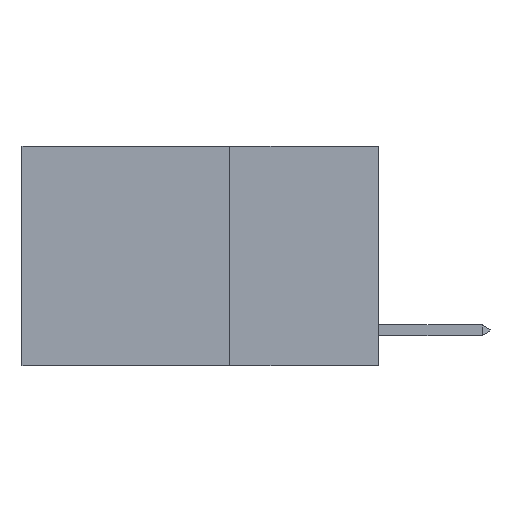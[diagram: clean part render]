
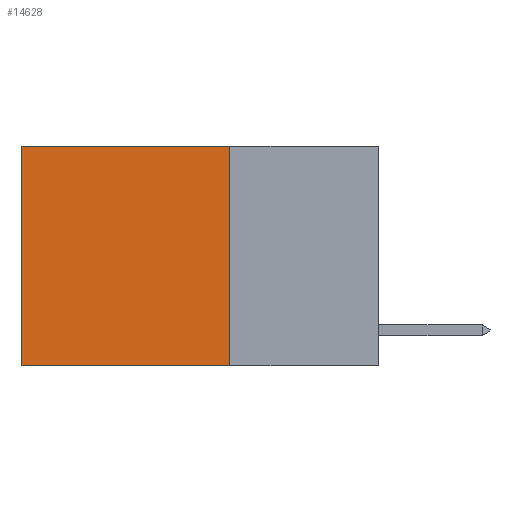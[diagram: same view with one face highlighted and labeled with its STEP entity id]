
A CAD part, left-side view. The second image highlights one B-rep face of the part: STEP entity #14628.
In plain terms, the highlighted planar face has unit normal (-1, 0, 0).
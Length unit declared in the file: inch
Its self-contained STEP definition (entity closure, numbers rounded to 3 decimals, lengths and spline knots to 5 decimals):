
#50 = CARTESIAN_POINT ( 'NONE',  ( 0.2625, 0.25, 0. ) ) ;
#1735 = EDGE_CURVE ( 'NONE', #9498, #5175, #27123, .T. ) ;
#2881 = ORIENTED_EDGE ( 'NONE', *, *, #27607, .F. ) ;
#4016 = EDGE_LOOP ( 'NONE', ( #20847, #16094, #2881, #5818 ) ) ;
#5175 = VERTEX_POINT ( 'NONE', #7162 ) ;
#5801 = CARTESIAN_POINT ( 'NONE',  ( 0.2625, 0.25, 0. ) ) ;
#5818 = ORIENTED_EDGE ( 'NONE', *, *, #21517, .T. ) ;
#5826 = EDGE_CURVE ( 'NONE', #18663, #5175, #27800, .T. ) ;
#7162 = CARTESIAN_POINT ( 'NONE',  ( 0.2625, 0.6, -0.37 ) ) ;
#7551 = DIRECTION ( 'NONE',  ( 0., 0., -1. ) ) ;
#7952 = PLANE ( 'NONE',  #23879 ) ;
#7965 = VERTEX_POINT ( 'NONE', #22360 ) ;
#9435 = VECTOR ( 'NONE', #19417, 39.37008 ) ;
#9498 = VERTEX_POINT ( 'NONE', #12818 ) ;
#9858 = CARTESIAN_POINT ( 'NONE',  ( 0.2625, 0.25, 0. ) ) ;
#10799 = LINE ( 'NONE', #50, #9435 ) ;
#11906 = CARTESIAN_POINT ( 'NONE',  ( 0.2625, 0.6, 0. ) ) ;
#12309 = DIRECTION ( 'NONE',  ( 0., 0., -1. ) ) ;
#12818 = CARTESIAN_POINT ( 'NONE',  ( 0.2625, 0.6, 0. ) ) ;
#14628 = ADVANCED_FACE ( 'NONE', ( #20873 ), #7952, .F. ) ;
#15901 = DIRECTION ( 'NONE',  ( 0., 1., 0. ) ) ;
#16094 = ORIENTED_EDGE ( 'NONE', *, *, #5826, .F. ) ;
#16362 = VECTOR ( 'NONE', #15901, 39.37008 ) ;
#16661 = CARTESIAN_POINT ( 'NONE',  ( 0.2625, 0.25, -0.37 ) ) ;
#18663 = VERTEX_POINT ( 'NONE', #16661 ) ;
#19417 = DIRECTION ( 'NONE',  ( 0., 1., 0. ) ) ;
#20014 = LINE ( 'NONE', #9858, #25781 ) ;
#20685 = VECTOR ( 'NONE', #7551, 39.37008 ) ;
#20847 = ORIENTED_EDGE ( 'NONE', *, *, #1735, .T. ) ;
#20873 = FACE_OUTER_BOUND ( 'NONE', #4016, .T. ) ;
#21517 = EDGE_CURVE ( 'NONE', #7965, #9498, #10799, .T. ) ;
#22360 = CARTESIAN_POINT ( 'NONE',  ( 0.2625, 0.25, 0. ) ) ;
#23879 = AXIS2_PLACEMENT_3D ( 'NONE', #5801, #25238, #12309 ) ;
#24960 = DIRECTION ( 'NONE',  ( 0., 0., -1. ) ) ;
#25238 = DIRECTION ( 'NONE',  ( 1., 0., 0. ) ) ;
#25781 = VECTOR ( 'NONE', #24960, 39.37008 ) ;
#26652 = CARTESIAN_POINT ( 'NONE',  ( 0.2625, 0.25, -0.37 ) ) ;
#27123 = LINE ( 'NONE', #11906, #20685 ) ;
#27607 = EDGE_CURVE ( 'NONE', #7965, #18663, #20014, .T. ) ;
#27800 = LINE ( 'NONE', #26652, #16362 ) ;
